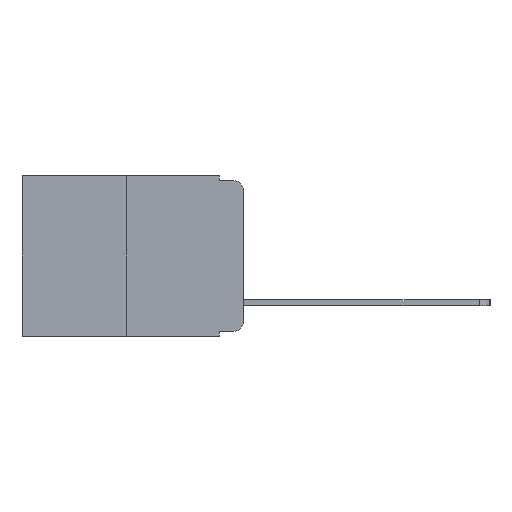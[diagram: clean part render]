
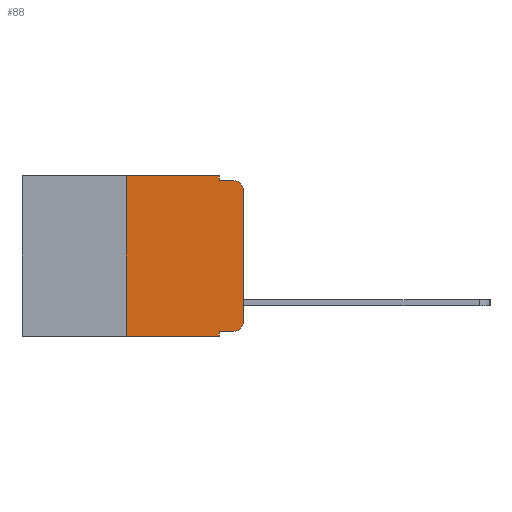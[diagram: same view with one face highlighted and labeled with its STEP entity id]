
A CAD part, left-side view. The second image highlights one B-rep face of the part: STEP entity #88.
In plain terms, the highlighted planar face has unit normal (-1, 0, 0).
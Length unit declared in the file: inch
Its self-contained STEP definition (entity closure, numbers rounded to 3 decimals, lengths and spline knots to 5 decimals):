
#25 = CARTESIAN_POINT ( 'NONE',  ( 0., 0.051, -0.333 ) ) ;
#88 = ADVANCED_FACE ( 'NONE', ( #5833 ), #5104, .F. ) ;
#92 = DIRECTION ( 'NONE',  ( 0., 0., -1. ) ) ;
#166 = VECTOR ( 'NONE', #305, 39.37008 ) ;
#181 = CARTESIAN_POINT ( 'NONE',  ( 0., 0.473, -0.343 ) ) ;
#305 = DIRECTION ( 'NONE',  ( 0., 0., 1. ) ) ;
#396 = EDGE_CURVE ( 'NONE', #9839, #2703, #11116, .T. ) ;
#647 = LINE ( 'NONE', #9829, #5739 ) ;
#752 = LINE ( 'NONE', #8493, #3186 ) ;
#985 = CARTESIAN_POINT ( 'NONE',  ( 0., 0.25, -0.343 ) ) ;
#1296 = EDGE_CURVE ( 'NONE', #9839, #4918, #4709, .T. ) ;
#1632 = VERTEX_POINT ( 'NONE', #9448 ) ;
#1671 = DIRECTION ( 'NONE',  ( 0., 0., -1. ) ) ;
#2121 = DIRECTION ( 'NONE',  ( 1., 0., 0. ) ) ;
#2125 = EDGE_CURVE ( 'NONE', #4918, #9563, #6791, .T. ) ;
#2389 = CARTESIAN_POINT ( 'NONE',  ( 0., 0.051, -0.343 ) ) ;
#2432 = VERTEX_POINT ( 'NONE', #9178 ) ;
#2682 = ORIENTED_EDGE ( 'NONE', *, *, #11849, .F. ) ;
#2703 = VERTEX_POINT ( 'NONE', #2389 ) ;
#2765 = ORIENTED_EDGE ( 'NONE', *, *, #11070, .F. ) ;
#2812 = AXIS2_PLACEMENT_3D ( 'NONE', #10194, #4568, #11065 ) ;
#2833 = ORIENTED_EDGE ( 'NONE', *, *, #10491, .F. ) ;
#2941 = EDGE_LOOP ( 'NONE', ( #4000, #3397, #2833, #2765, #2682, #10174, #8009, #7869, #7816, #7614 ) ) ;
#3186 = VECTOR ( 'NONE', #3698, 39.37008 ) ;
#3188 = EDGE_CURVE ( 'NONE', #3477, #2703, #5429, .T. ) ;
#3397 = ORIENTED_EDGE ( 'NONE', *, *, #9898, .T. ) ;
#3477 = VERTEX_POINT ( 'NONE', #985 ) ;
#3582 = AXIS2_PLACEMENT_3D ( 'NONE', #11846, #11922, #92 ) ;
#3698 = DIRECTION ( 'NONE',  ( 0., 0., -1. ) ) ;
#3705 = VERTEX_POINT ( 'NONE', #7470 ) ;
#4000 = ORIENTED_EDGE ( 'NONE', *, *, #9318, .T. ) ;
#4220 = CARTESIAN_POINT ( 'NONE',  ( 0., 0.473, 0. ) ) ;
#4512 = VECTOR ( 'NONE', #10778, 39.37008 ) ;
#4568 = DIRECTION ( 'NONE',  ( -1., 0., 0. ) ) ;
#4709 = LINE ( 'NONE', #25, #10004 ) ;
#4759 = VERTEX_POINT ( 'NONE', #8102 ) ;
#4832 = AXIS2_PLACEMENT_3D ( 'NONE', #10752, #2121, #1671 ) ;
#4918 = VERTEX_POINT ( 'NONE', #8279 ) ;
#5104 = PLANE ( 'NONE',  #4832 ) ;
#5207 = LINE ( 'NONE', #10644, #9900 ) ;
#5429 = LINE ( 'NONE', #181, #12637 ) ;
#5739 = VECTOR ( 'NONE', #7091, 39.37008 ) ;
#5833 = FACE_OUTER_BOUND ( 'NONE', #2941, .T. ) ;
#5989 = DIRECTION ( 'NONE',  ( 0., -1., 0. ) ) ;
#5993 = LINE ( 'NONE', #10421, #166 ) ;
#6289 = CIRCLE ( 'NONE', #2812, 0.02 ) ;
#6791 = CIRCLE ( 'NONE', #3582, 0.02 ) ;
#7027 = DIRECTION ( 'NONE',  ( 0., -1., 0. ) ) ;
#7086 = LINE ( 'NONE', #4220, #4512 ) ;
#7091 = DIRECTION ( 'NONE',  ( 0., 0., 1. ) ) ;
#7118 = CARTESIAN_POINT ( 'NONE',  ( 0., 0., -0.313 ) ) ;
#7406 = CARTESIAN_POINT ( 'NONE',  ( 0., 0.051, -0.333 ) ) ;
#7470 = CARTESIAN_POINT ( 'NONE',  ( 0., 0.051, 0. ) ) ;
#7600 = DIRECTION ( 'NONE',  ( 0., -1., 0. ) ) ;
#7614 = ORIENTED_EDGE ( 'NONE', *, *, #2125, .T. ) ;
#7816 = ORIENTED_EDGE ( 'NONE', *, *, #1296, .T. ) ;
#7869 = ORIENTED_EDGE ( 'NONE', *, *, #396, .F. ) ;
#8009 = ORIENTED_EDGE ( 'NONE', *, *, #3188, .T. ) ;
#8102 = CARTESIAN_POINT ( 'NONE',  ( 0., 0.25, 0. ) ) ;
#8279 = CARTESIAN_POINT ( 'NONE',  ( 0., 0.02, -0.333 ) ) ;
#8470 = VERTEX_POINT ( 'NONE', #10573 ) ;
#8493 = CARTESIAN_POINT ( 'NONE',  ( 0., 0.051, 0. ) ) ;
#9178 = CARTESIAN_POINT ( 'NONE',  ( 0., 0., -0.03 ) ) ;
#9318 = EDGE_CURVE ( 'NONE', #9563, #2432, #5993, .T. ) ;
#9448 = CARTESIAN_POINT ( 'NONE',  ( 0., 0.051, -0.01 ) ) ;
#9563 = VERTEX_POINT ( 'NONE', #7118 ) ;
#9829 = CARTESIAN_POINT ( 'NONE',  ( 0., 0.25, 0. ) ) ;
#9839 = VERTEX_POINT ( 'NONE', #7406 ) ;
#9898 = EDGE_CURVE ( 'NONE', #2432, #8470, #6289, .T. ) ;
#9900 = VECTOR ( 'NONE', #7027, 39.37008 ) ;
#10004 = VECTOR ( 'NONE', #5989, 39.37008 ) ;
#10174 = ORIENTED_EDGE ( 'NONE', *, *, #11612, .F. ) ;
#10194 = CARTESIAN_POINT ( 'NONE',  ( 0., 0.02, -0.03 ) ) ;
#10421 = CARTESIAN_POINT ( 'NONE',  ( 0., 0., 0. ) ) ;
#10491 = EDGE_CURVE ( 'NONE', #1632, #8470, #5207, .T. ) ;
#10573 = CARTESIAN_POINT ( 'NONE',  ( 0., 0.02, -0.01 ) ) ;
#10644 = CARTESIAN_POINT ( 'NONE',  ( 0., 0.051, -0.01 ) ) ;
#10752 = CARTESIAN_POINT ( 'NONE',  ( 0., 0.473, 0. ) ) ;
#10778 = DIRECTION ( 'NONE',  ( 0., -1., 0. ) ) ;
#10842 = VECTOR ( 'NONE', #11680, 39.37008 ) ;
#11065 = DIRECTION ( 'NONE',  ( 0., 0., -1. ) ) ;
#11070 = EDGE_CURVE ( 'NONE', #3705, #1632, #752, .T. ) ;
#11116 = LINE ( 'NONE', #11168, #10842 ) ;
#11168 = CARTESIAN_POINT ( 'NONE',  ( 0., 0.051, 0. ) ) ;
#11612 = EDGE_CURVE ( 'NONE', #3477, #4759, #647, .T. ) ;
#11680 = DIRECTION ( 'NONE',  ( 0., 0., -1. ) ) ;
#11846 = CARTESIAN_POINT ( 'NONE',  ( 0., 0.02, -0.313 ) ) ;
#11849 = EDGE_CURVE ( 'NONE', #4759, #3705, #7086, .T. ) ;
#11922 = DIRECTION ( 'NONE',  ( -1., 0., 0. ) ) ;
#12637 = VECTOR ( 'NONE', #7600, 39.37008 ) ;
